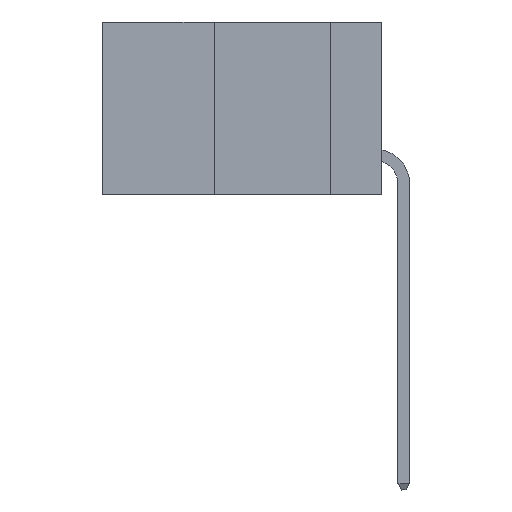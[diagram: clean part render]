
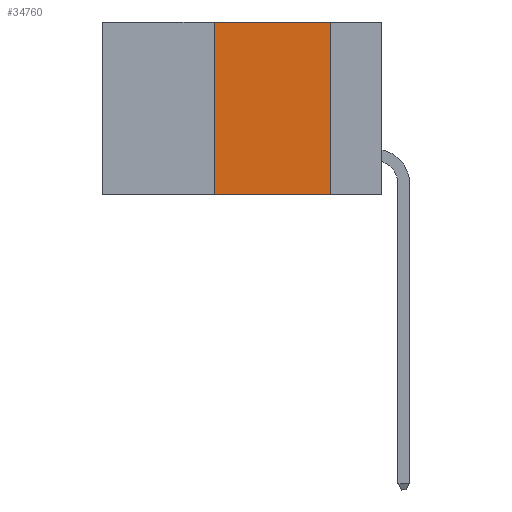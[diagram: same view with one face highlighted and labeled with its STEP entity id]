
A CAD part, left-side view. The second image highlights one B-rep face of the part: STEP entity #34760.
In plain terms, the highlighted planar face has unit normal (-1, 0, 0).
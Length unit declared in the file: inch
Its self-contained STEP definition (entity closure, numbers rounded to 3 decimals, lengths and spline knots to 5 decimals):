
#78 = VERTEX_POINT ( 'NONE', #30328 ) ;
#2211 = ORIENTED_EDGE ( 'NONE', *, *, #27033, .F. ) ;
#3895 = DIRECTION ( 'NONE',  ( 0., 0., -1. ) ) ;
#7112 = ORIENTED_EDGE ( 'NONE', *, *, #9938, .T. ) ;
#7938 = EDGE_CURVE ( 'NONE', #31119, #26058, #27669, .T. ) ;
#8214 = CARTESIAN_POINT ( 'NONE',  ( 0., 0.11, 0. ) ) ;
#8715 = ORIENTED_EDGE ( 'NONE', *, *, #24038, .F. ) ;
#9938 = EDGE_CURVE ( 'NONE', #13853, #26058, #14661, .T. ) ;
#10144 = CARTESIAN_POINT ( 'NONE',  ( 0., 0.36, 0. ) ) ;
#10895 = DIRECTION ( 'NONE',  ( 0., 0., -1. ) ) ;
#11559 = EDGE_LOOP ( 'NONE', ( #14375, #8715, #2211, #7112 ) ) ;
#11592 = DIRECTION ( 'NONE',  ( 0., -1., 0. ) ) ;
#12254 = CARTESIAN_POINT ( 'NONE',  ( 0., 0.6, 0. ) ) ;
#12960 = CARTESIAN_POINT ( 'NONE',  ( 0., 0.6, -0.37 ) ) ;
#13438 = DIRECTION ( 'NONE',  ( 0., 0., 1. ) ) ;
#13853 = VERTEX_POINT ( 'NONE', #18384 ) ;
#14303 = FACE_OUTER_BOUND ( 'NONE', #11559, .T. ) ;
#14375 = ORIENTED_EDGE ( 'NONE', *, *, #7938, .F. ) ;
#14661 = LINE ( 'NONE', #12960, #34880 ) ;
#18384 = CARTESIAN_POINT ( 'NONE',  ( 0., 0.36, -0.37 ) ) ;
#18833 = CARTESIAN_POINT ( 'NONE',  ( 0., 0.11, 0. ) ) ;
#20122 = AXIS2_PLACEMENT_3D ( 'NONE', #12254, #31165, #3895 ) ;
#22716 = CARTESIAN_POINT ( 'NONE',  ( 0., 0.6, 0. ) ) ;
#24038 = EDGE_CURVE ( 'NONE', #78, #31119, #31178, .T. ) ;
#26058 = VERTEX_POINT ( 'NONE', #32787 ) ;
#26440 = DIRECTION ( 'NONE',  ( 0., -1., 0. ) ) ;
#27033 = EDGE_CURVE ( 'NONE', #13853, #78, #34737, .T. ) ;
#27149 = VECTOR ( 'NONE', #13438, 39.37008 ) ;
#27669 = LINE ( 'NONE', #18833, #30608 ) ;
#28454 = PLANE ( 'NONE',  #20122 ) ;
#30328 = CARTESIAN_POINT ( 'NONE',  ( 0., 0.36, 0. ) ) ;
#30608 = VECTOR ( 'NONE', #10895, 39.37008 ) ;
#31119 = VERTEX_POINT ( 'NONE', #8214 ) ;
#31165 = DIRECTION ( 'NONE',  ( 1., 0., 0. ) ) ;
#31178 = LINE ( 'NONE', #22716, #34146 ) ;
#32787 = CARTESIAN_POINT ( 'NONE',  ( 0., 0.11, -0.37 ) ) ;
#34146 = VECTOR ( 'NONE', #11592, 39.37008 ) ;
#34737 = LINE ( 'NONE', #10144, #27149 ) ;
#34760 = ADVANCED_FACE ( 'NONE', ( #14303 ), #28454, .F. ) ;
#34880 = VECTOR ( 'NONE', #26440, 39.37008 ) ;
